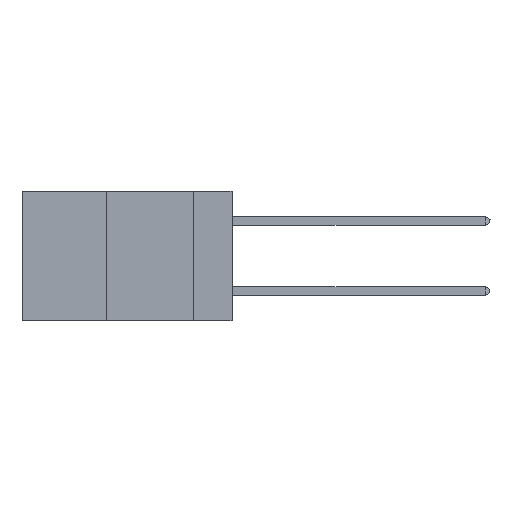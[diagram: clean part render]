
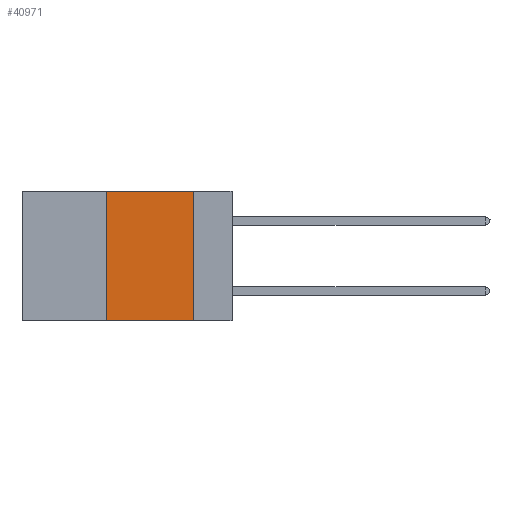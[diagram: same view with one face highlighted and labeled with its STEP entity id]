
A CAD part, left-side view. The second image highlights one B-rep face of the part: STEP entity #40971.
In plain terms, the highlighted planar face has unit normal (-1, 0, 0).
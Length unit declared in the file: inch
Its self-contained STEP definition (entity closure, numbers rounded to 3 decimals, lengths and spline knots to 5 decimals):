
#5114 = DIRECTION ( 'NONE',  ( 0., 0., -1. ) ) ;
#6253 = CARTESIAN_POINT ( 'NONE',  ( 0., 0.11, -0.37 ) ) ;
#6529 = EDGE_CURVE ( 'NONE', #22265, #34284, #27921, .T. ) ;
#6598 = CARTESIAN_POINT ( 'NONE',  ( 0., 0.11, 0. ) ) ;
#8513 = ORIENTED_EDGE ( 'NONE', *, *, #6529, .F. ) ;
#9249 = LINE ( 'NONE', #37280, #42521 ) ;
#10372 = DIRECTION ( 'NONE',  ( 0., -1., 0. ) ) ;
#11215 = ORIENTED_EDGE ( 'NONE', *, *, #27435, .F. ) ;
#11510 = CARTESIAN_POINT ( 'NONE',  ( 0., 0.6, 0. ) ) ;
#14422 = CARTESIAN_POINT ( 'NONE',  ( 0., 0.36, 0. ) ) ;
#15377 = PLANE ( 'NONE',  #30103 ) ;
#15607 = CARTESIAN_POINT ( 'NONE',  ( 0., 0.36, -0.37 ) ) ;
#16485 = VECTOR ( 'NONE', #34451, 39.37008 ) ;
#17149 = CARTESIAN_POINT ( 'NONE',  ( 0., 0.6, -0.37 ) ) ;
#17532 = LINE ( 'NONE', #6598, #33904 ) ;
#20281 = EDGE_CURVE ( 'NONE', #44935, #22265, #9249, .T. ) ;
#21276 = ORIENTED_EDGE ( 'NONE', *, *, #20281, .F. ) ;
#22265 = VERTEX_POINT ( 'NONE', #14422 ) ;
#27198 = EDGE_LOOP ( 'NONE', ( #11215, #8513, #21276, #33242 ) ) ;
#27435 = EDGE_CURVE ( 'NONE', #34284, #38351, #17532, .T. ) ;
#27921 = LINE ( 'NONE', #38176, #35935 ) ;
#28212 = EDGE_CURVE ( 'NONE', #44935, #38351, #38336, .T. ) ;
#29295 = DIRECTION ( 'NONE',  ( 1., 0., 0. ) ) ;
#30103 = AXIS2_PLACEMENT_3D ( 'NONE', #11510, #29295, #5114 ) ;
#33242 = ORIENTED_EDGE ( 'NONE', *, *, #28212, .T. ) ;
#33620 = DIRECTION ( 'NONE',  ( 0., 0., 1. ) ) ;
#33904 = VECTOR ( 'NONE', #34392, 39.37008 ) ;
#34058 = CARTESIAN_POINT ( 'NONE',  ( 0., 0.11, 0. ) ) ;
#34284 = VERTEX_POINT ( 'NONE', #34058 ) ;
#34392 = DIRECTION ( 'NONE',  ( 0., 0., -1. ) ) ;
#34451 = DIRECTION ( 'NONE',  ( 0., -1., 0. ) ) ;
#35935 = VECTOR ( 'NONE', #10372, 39.37008 ) ;
#37280 = CARTESIAN_POINT ( 'NONE',  ( 0., 0.36, 0. ) ) ;
#38176 = CARTESIAN_POINT ( 'NONE',  ( 0., 0.6, 0. ) ) ;
#38336 = LINE ( 'NONE', #17149, #16485 ) ;
#38351 = VERTEX_POINT ( 'NONE', #6253 ) ;
#40971 = ADVANCED_FACE ( 'NONE', ( #42732 ), #15377, .F. ) ;
#42521 = VECTOR ( 'NONE', #33620, 39.37008 ) ;
#42732 = FACE_OUTER_BOUND ( 'NONE', #27198, .T. ) ;
#44935 = VERTEX_POINT ( 'NONE', #15607 ) ;
